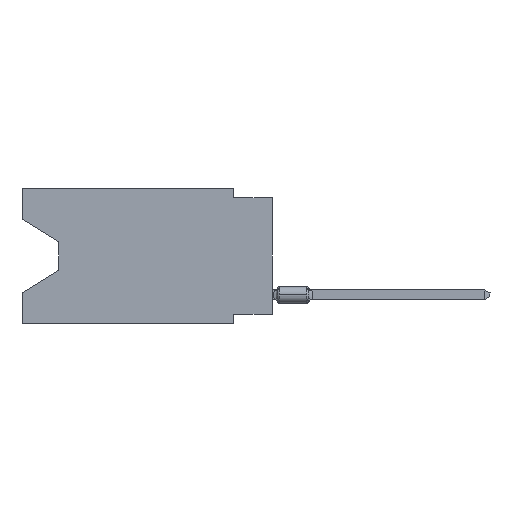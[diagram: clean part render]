
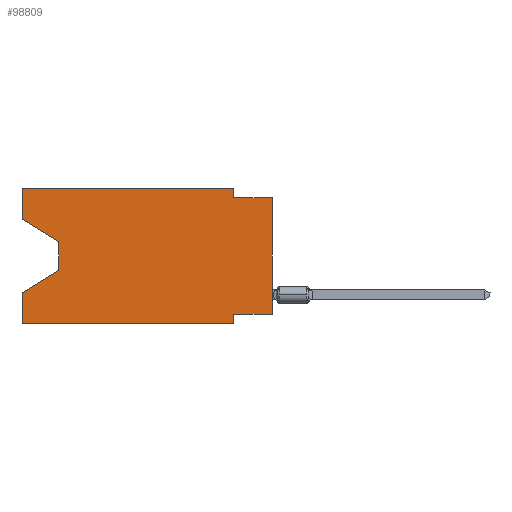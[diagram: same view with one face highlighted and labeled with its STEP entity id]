
A CAD part, left-side view. The second image highlights one B-rep face of the part: STEP entity #98809.
In plain terms, the highlighted planar face has unit normal (-1, 0, 0).
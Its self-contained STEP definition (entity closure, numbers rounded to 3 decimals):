
#2468 = VECTOR ( 'NONE', #110151, 1000. ) ;
#3712 = VERTEX_POINT ( 'NONE', #13057 ) ;
#4911 = CARTESIAN_POINT ( 'NONE',  ( 0., 16.383, -8.89 ) ) ;
#5820 = VECTOR ( 'NONE', #50466, 1000. ) ;
#8879 = CARTESIAN_POINT ( 'NONE',  ( 0., 16.383, -2.038 ) ) ;
#12316 = EDGE_CURVE ( 'NONE', #82385, #76280, #73180, .T. ) ;
#12807 = ORIENTED_EDGE ( 'NONE', *, *, #33519, .F. ) ;
#13052 = LINE ( 'NONE', #49381, #112484 ) ;
#13057 = CARTESIAN_POINT ( 'NONE',  ( 0., 16.383, -6.852 ) ) ;
#13774 = VERTEX_POINT ( 'NONE', #32214 ) ;
#13986 = DIRECTION ( 'NONE',  ( 1., 0., 0. ) ) ;
#14065 = LINE ( 'NONE', #87311, #107928 ) ;
#14143 = CARTESIAN_POINT ( 'NONE',  ( 0., 2.54, -8.89 ) ) ;
#14344 = CARTESIAN_POINT ( 'NONE',  ( 0., 16.383, -2.038 ) ) ;
#15451 = EDGE_CURVE ( 'NONE', #82044, #90404, #13052, .T. ) ;
#16006 = ORIENTED_EDGE ( 'NONE', *, *, #57987, .F. ) ;
#20128 = VERTEX_POINT ( 'NONE', #96188 ) ;
#20709 = DIRECTION ( 'NONE',  ( 0., -1., 0. ) ) ;
#23134 = CARTESIAN_POINT ( 'NONE',  ( 0., 16.383, 0. ) ) ;
#25153 = VECTOR ( 'NONE', #20709, 1000. ) ;
#26754 = EDGE_CURVE ( 'NONE', #41388, #76280, #14065, .T. ) ;
#27393 = ORIENTED_EDGE ( 'NONE', *, *, #95201, .T. ) ;
#28171 = CARTESIAN_POINT ( 'NONE',  ( 0., 16.383, -8.89 ) ) ;
#30621 = EDGE_CURVE ( 'NONE', #69597, #40506, #109790, .T. ) ;
#30677 = CARTESIAN_POINT ( 'NONE',  ( 0., 16.383, 0. ) ) ;
#30976 = ORIENTED_EDGE ( 'NONE', *, *, #31360, .F. ) ;
#31360 = EDGE_CURVE ( 'NONE', #20128, #82385, #81355, .T. ) ;
#31696 = ORIENTED_EDGE ( 'NONE', *, *, #116957, .F. ) ;
#31851 = FACE_OUTER_BOUND ( 'NONE', #89439, .T. ) ;
#32214 = CARTESIAN_POINT ( 'NONE',  ( 0., 16.383, 0. ) ) ;
#33519 = EDGE_CURVE ( 'NONE', #69597, #3712, #97570, .T. ) ;
#33889 = EDGE_CURVE ( 'NONE', #90404, #3712, #77789, .T. ) ;
#40323 = CARTESIAN_POINT ( 'NONE',  ( 0., 16.383, 0. ) ) ;
#40506 = VERTEX_POINT ( 'NONE', #108537 ) ;
#41388 = VERTEX_POINT ( 'NONE', #73663 ) ;
#41941 = VERTEX_POINT ( 'NONE', #14344 ) ;
#45037 = CARTESIAN_POINT ( 'NONE',  ( 0., 2.54, 0. ) ) ;
#45722 = ORIENTED_EDGE ( 'NONE', *, *, #76947, .F. ) ;
#47393 = LINE ( 'NONE', #83708, #101626 ) ;
#49381 = CARTESIAN_POINT ( 'NONE',  ( 0., 13.97, -3.505 ) ) ;
#50392 = DIRECTION ( 'NONE',  ( 0., 0., 1. ) ) ;
#50466 = DIRECTION ( 'NONE',  ( 0., 0., -1. ) ) ;
#51650 = CARTESIAN_POINT ( 'NONE',  ( 0., 2.54, -8.255 ) ) ;
#52161 = CARTESIAN_POINT ( 'NONE',  ( 0., 13.97, -5.385 ) ) ;
#53375 = DIRECTION ( 'NONE',  ( 0., 0., -1. ) ) ;
#54176 = LINE ( 'NONE', #8879, #2468 ) ;
#57527 = VECTOR ( 'NONE', #64492, 1000. ) ;
#57857 = VECTOR ( 'NONE', #114879, 1000. ) ;
#57987 = EDGE_CURVE ( 'NONE', #41388, #68954, #67362, .T. ) ;
#58070 = PLANE ( 'NONE',  #115327 ) ;
#60741 = CARTESIAN_POINT ( 'NONE',  ( 0., 13.97, -3.505 ) ) ;
#63151 = ORIENTED_EDGE ( 'NONE', *, *, #12316, .F. ) ;
#64492 = DIRECTION ( 'NONE',  ( 0., -1., 0. ) ) ;
#66764 = DIRECTION ( 'NONE',  ( 0., 1., 0. ) ) ;
#67009 = DIRECTION ( 'NONE',  ( 0., 0., -1. ) ) ;
#67362 = LINE ( 'NONE', #67946, #98010 ) ;
#67946 = CARTESIAN_POINT ( 'NONE',  ( 0., 0., -8.255 ) ) ;
#68954 = VERTEX_POINT ( 'NONE', #51650 ) ;
#69597 = VERTEX_POINT ( 'NONE', #4911 ) ;
#69660 = CARTESIAN_POINT ( 'NONE',  ( 0., 0., -0.635 ) ) ;
#73180 = LINE ( 'NONE', #109512, #25153 ) ;
#73663 = CARTESIAN_POINT ( 'NONE',  ( 0., 0., -8.255 ) ) ;
#76280 = VERTEX_POINT ( 'NONE', #69660 ) ;
#76913 = VECTOR ( 'NONE', #115896, 1000. ) ;
#76947 = EDGE_CURVE ( 'NONE', #13774, #20128, #47393, .T. ) ;
#77789 = LINE ( 'NONE', #52161, #76913 ) ;
#78651 = CARTESIAN_POINT ( 'NONE',  ( 0., 13.97, -5.385 ) ) ;
#79876 = ORIENTED_EDGE ( 'NONE', *, *, #26754, .T. ) ;
#80313 = VECTOR ( 'NONE', #53375, 1000. ) ;
#81355 = LINE ( 'NONE', #45037, #80313 ) ;
#82044 = VERTEX_POINT ( 'NONE', #60741 ) ;
#82385 = VERTEX_POINT ( 'NONE', #92237 ) ;
#83708 = CARTESIAN_POINT ( 'NONE',  ( 0., 16.383, 0. ) ) ;
#85714 = DIRECTION ( 'NONE',  ( 0., 0., -1. ) ) ;
#87311 = CARTESIAN_POINT ( 'NONE',  ( 0., 0., 0. ) ) ;
#87669 = ORIENTED_EDGE ( 'NONE', *, *, #15451, .T. ) ;
#87936 = EDGE_CURVE ( 'NONE', #68954, #40506, #95740, .T. ) ;
#89439 = EDGE_LOOP ( 'NONE', ( #27393, #87669, #96385, #12807, #89752, #105713, #16006, #79876, #63151, #30976, #45722, #31696 ) ) ;
#89752 = ORIENTED_EDGE ( 'NONE', *, *, #30621, .T. ) ;
#90404 = VERTEX_POINT ( 'NONE', #78651 ) ;
#92237 = CARTESIAN_POINT ( 'NONE',  ( 0., 2.54, -0.635 ) ) ;
#93247 = DIRECTION ( 'NONE',  ( 0., -1., 0. ) ) ;
#95201 = EDGE_CURVE ( 'NONE', #41941, #82044, #54176, .T. ) ;
#95740 = LINE ( 'NONE', #14143, #5820 ) ;
#96188 = CARTESIAN_POINT ( 'NONE',  ( 0., 2.54, 0. ) ) ;
#96385 = ORIENTED_EDGE ( 'NONE', *, *, #33889, .T. ) ;
#97464 = LINE ( 'NONE', #40323, #110408 ) ;
#97570 = LINE ( 'NONE', #23134, #57857 ) ;
#98010 = VECTOR ( 'NONE', #66764, 1000. ) ;
#98809 = ADVANCED_FACE ( 'NONE', ( #31851 ), #58070, .F. ) ;
#101626 = VECTOR ( 'NONE', #93247, 1000. ) ;
#105713 = ORIENTED_EDGE ( 'NONE', *, *, #87936, .F. ) ;
#107928 = VECTOR ( 'NONE', #50392, 1000. ) ;
#108537 = CARTESIAN_POINT ( 'NONE',  ( 0., 2.54, -8.89 ) ) ;
#109336 = DIRECTION ( 'NONE',  ( 0., 0., 1. ) ) ;
#109512 = CARTESIAN_POINT ( 'NONE',  ( 0., 0., -0.635 ) ) ;
#109790 = LINE ( 'NONE', #28171, #57527 ) ;
#110151 = DIRECTION ( 'NONE',  ( 0., -0.855, -0.519 ) ) ;
#110408 = VECTOR ( 'NONE', #109336, 1000. ) ;
#112484 = VECTOR ( 'NONE', #85714, 1000. ) ;
#114879 = DIRECTION ( 'NONE',  ( 0., 0., 1. ) ) ;
#115327 = AXIS2_PLACEMENT_3D ( 'NONE', #30677, #13986, #67009 ) ;
#115896 = DIRECTION ( 'NONE',  ( 0., 0.855, -0.519 ) ) ;
#116957 = EDGE_CURVE ( 'NONE', #41941, #13774, #97464, .T. ) ;
